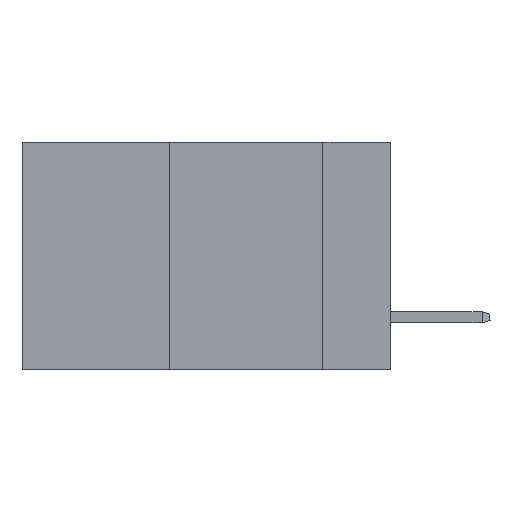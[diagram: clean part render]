
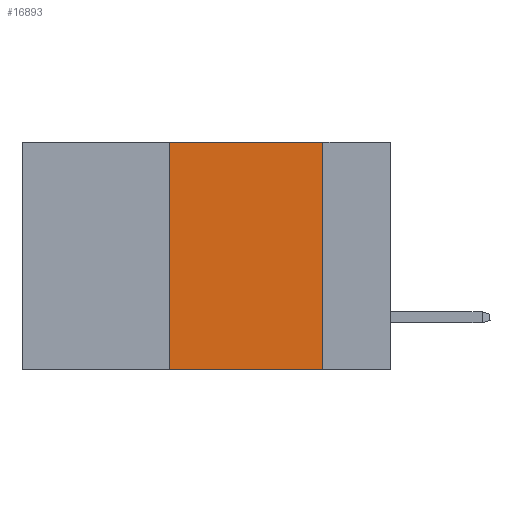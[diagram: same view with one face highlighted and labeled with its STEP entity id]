
A CAD part, left-side view. The second image highlights one B-rep face of the part: STEP entity #16893.
In plain terms, the highlighted planar face has unit normal (-1, 0, 0).
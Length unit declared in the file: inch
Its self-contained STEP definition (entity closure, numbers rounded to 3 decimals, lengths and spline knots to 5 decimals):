
#347 = ORIENTED_EDGE ( 'NONE', *, *, #12163, .F. ) ;
#686 = LINE ( 'NONE', #5971, #8610 ) ;
#1797 = EDGE_LOOP ( 'NONE', ( #347, #3574, #7698, #17885 ) ) ;
#2891 = VECTOR ( 'NONE', #5035, 39.37008 ) ;
#2931 = AXIS2_PLACEMENT_3D ( 'NONE', #10990, #10622, #6405 ) ;
#3329 = DIRECTION ( 'NONE',  ( 0., 0., -1. ) ) ;
#3574 = ORIENTED_EDGE ( 'NONE', *, *, #9970, .F. ) ;
#3583 = PLANE ( 'NONE',  #2931 ) ;
#4201 = VERTEX_POINT ( 'NONE', #7334 ) ;
#4670 = LINE ( 'NONE', #7257, #6647 ) ;
#5035 = DIRECTION ( 'NONE',  ( 0., 0., 1. ) ) ;
#5971 = CARTESIAN_POINT ( 'NONE',  ( 0., 0.11, 0. ) ) ;
#6405 = DIRECTION ( 'NONE',  ( 0., 0., -1. ) ) ;
#6515 = CARTESIAN_POINT ( 'NONE',  ( 0., 0.36, 0. ) ) ;
#6647 = VECTOR ( 'NONE', #14404, 39.37008 ) ;
#6649 = LINE ( 'NONE', #6515, #2891 ) ;
#6906 = DIRECTION ( 'NONE',  ( 0., -1., 0. ) ) ;
#6994 = CARTESIAN_POINT ( 'NONE',  ( 0., 0.36, 0. ) ) ;
#7257 = CARTESIAN_POINT ( 'NONE',  ( 0., 0.6, -0.37 ) ) ;
#7334 = CARTESIAN_POINT ( 'NONE',  ( 0., 0.11, -0.37 ) ) ;
#7698 = ORIENTED_EDGE ( 'NONE', *, *, #11467, .F. ) ;
#8167 = CARTESIAN_POINT ( 'NONE',  ( 0., 0.11, 0. ) ) ;
#8372 = VERTEX_POINT ( 'NONE', #6994 ) ;
#8610 = VECTOR ( 'NONE', #3329, 39.37008 ) ;
#8702 = CARTESIAN_POINT ( 'NONE',  ( 0., 0.36, -0.37 ) ) ;
#9970 = EDGE_CURVE ( 'NONE', #8372, #10625, #16517, .T. ) ;
#10622 = DIRECTION ( 'NONE',  ( 1., 0., 0. ) ) ;
#10625 = VERTEX_POINT ( 'NONE', #8167 ) ;
#10990 = CARTESIAN_POINT ( 'NONE',  ( 0., 0.6, 0. ) ) ;
#11467 = EDGE_CURVE ( 'NONE', #15427, #8372, #6649, .T. ) ;
#11665 = FACE_OUTER_BOUND ( 'NONE', #1797, .T. ) ;
#12163 = EDGE_CURVE ( 'NONE', #10625, #4201, #686, .T. ) ;
#13052 = VECTOR ( 'NONE', #6906, 39.37008 ) ;
#14404 = DIRECTION ( 'NONE',  ( 0., -1., 0. ) ) ;
#15427 = VERTEX_POINT ( 'NONE', #8702 ) ;
#16372 = EDGE_CURVE ( 'NONE', #15427, #4201, #4670, .T. ) ;
#16517 = LINE ( 'NONE', #18155, #13052 ) ;
#16893 = ADVANCED_FACE ( 'NONE', ( #11665 ), #3583, .F. ) ;
#17885 = ORIENTED_EDGE ( 'NONE', *, *, #16372, .T. ) ;
#18155 = CARTESIAN_POINT ( 'NONE',  ( 0., 0.6, 0. ) ) ;
